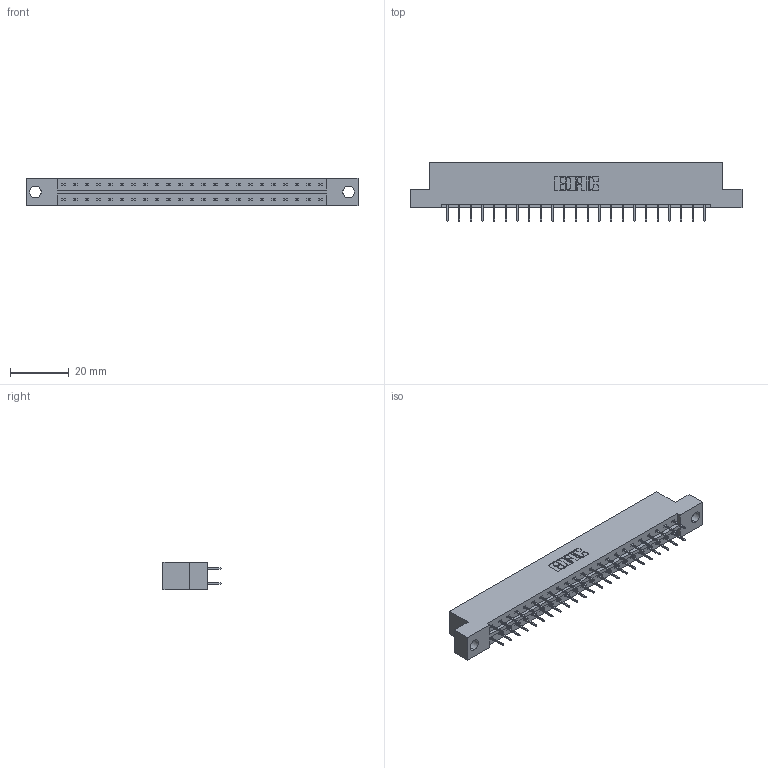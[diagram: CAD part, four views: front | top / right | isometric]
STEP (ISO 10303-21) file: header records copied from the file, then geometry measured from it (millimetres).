
FILE_DESCRIPTION (( 'STEP AP203' ), '1' );
FILE_NAME ('333-046-524-204.STEP', '2018-08-03T22:14:52', ( '' ), ( '' ), 'SwSTEP 2.0', 'SolidWorks 2016', '' );
FILE_SCHEMA (( 'CONFIG_CONTROL_DESIGN' ));
Length unit declared in the file: inch
Products named in the file (3): 345-292-001_345-293-124; 333-046-524-204; 333 Part_Flush - .156 Dia - TH
Assembly tree (47 placements, depth 2):
  333-046-524-204
    333 Part_Flush - .156 Dia - TH
    345-292-001_345-293-124  x46
Bounding box: 112.67 x 19.69 x 9.4 mm (x, y, z)
Volume: 11168.3 mm3; surface area: 12590 mm2
Topology: 47 solids, 47 shells, 2690 faces, 7625 edges, 4898 vertices
Faces by surface type: plane 2002, cylinder 688
Entity records: 17331 total; most frequent: CARTESIAN_POINT 2894, ORIENTED_EDGE 2830, DIRECTION 2507, EDGE_CURVE 1415, VECTOR 1291, LINE 1291, VERTEX_POINT 938, AXIS2_PLACEMENT_3D 608
